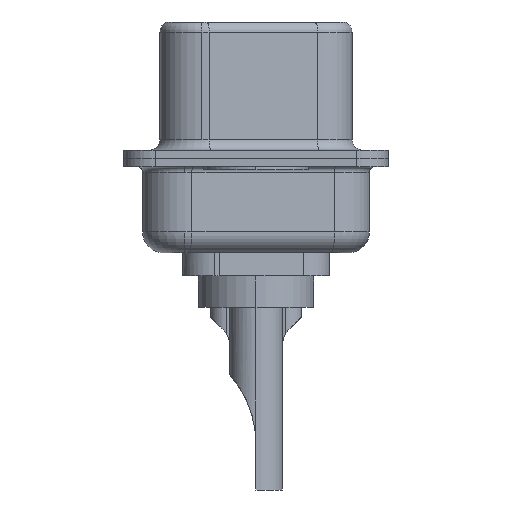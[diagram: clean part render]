
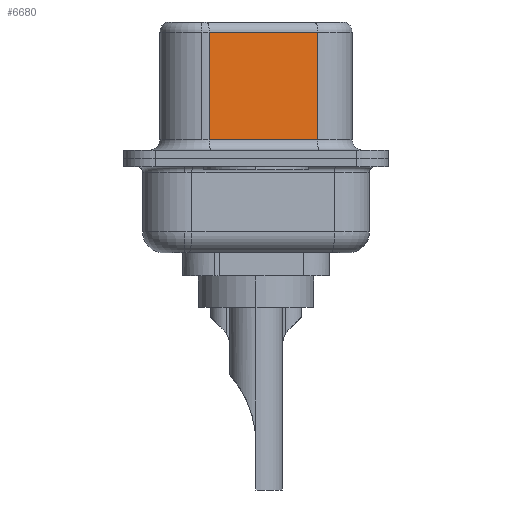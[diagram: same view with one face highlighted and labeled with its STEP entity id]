
A CAD part, left-side view. The second image highlights one B-rep face of the part: STEP entity #6680.
In plain terms, the highlighted planar face has unit normal (-0.985, -0.174, 0).
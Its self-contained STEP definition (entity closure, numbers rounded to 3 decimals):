
#112 = DIRECTION ( 'NONE',  ( 0.174, -0.985, 0. ) ) ;
#612 = DIRECTION ( 'NONE',  ( 0., 0., -1. ) ) ;
#1322 = CARTESIAN_POINT ( 'NONE',  ( 4.585, -2.927, 0.9 ) ) ;
#1980 = LINE ( 'NONE', #2978, #8455 ) ;
#2912 = DIRECTION ( 'NONE',  ( 0., 0., -1. ) ) ;
#2978 = CARTESIAN_POINT ( 'NONE',  ( 4.585, -2.927, 6.52 ) ) ;
#3822 = DIRECTION ( 'NONE',  ( -0.174, 0.985, 0. ) ) ;
#5234 = FACE_OUTER_BOUND ( 'NONE', #12017, .T. ) ;
#5388 = CARTESIAN_POINT ( 'NONE',  ( 3.675, 2.233, 6.52 ) ) ;
#5440 = ORIENTED_EDGE ( 'NONE', *, *, #6648, .T. ) ;
#6086 = VECTOR ( 'NONE', #3822, 1000. ) ;
#6648 = EDGE_CURVE ( 'NONE', #10150, #11646, #12345, .T. ) ;
#6673 = DIRECTION ( 'NONE',  ( 0.985, 0.174, 0. ) ) ;
#6680 = ADVANCED_FACE ( 'NONE', ( #5234 ), #11411, .F. ) ;
#6693 = EDGE_CURVE ( 'NONE', #13265, #9783, #1980, .T. ) ;
#7518 = CARTESIAN_POINT ( 'NONE',  ( 4.585, -2.927, 6.02 ) ) ;
#7602 = CARTESIAN_POINT ( 'NONE',  ( 4.585, -2.927, 0.9 ) ) ;
#8455 = VECTOR ( 'NONE', #612, 1000. ) ;
#9783 = VERTEX_POINT ( 'NONE', #7602 ) ;
#9978 = LINE ( 'NONE', #7518, #6086 ) ;
#10150 = VERTEX_POINT ( 'NONE', #14255 ) ;
#10217 = CARTESIAN_POINT ( 'NONE',  ( 4.585, -2.927, 6.52 ) ) ;
#10387 = ORIENTED_EDGE ( 'NONE', *, *, #6693, .F. ) ;
#10390 = ORIENTED_EDGE ( 'NONE', *, *, #12658, .T. ) ;
#10745 = ORIENTED_EDGE ( 'NONE', *, *, #11392, .T. ) ;
#11392 = EDGE_CURVE ( 'NONE', #11646, #9783, #13777, .T. ) ;
#11411 = PLANE ( 'NONE',  #14579 ) ;
#11542 = CARTESIAN_POINT ( 'NONE',  ( 4.585, -2.927, 6.02 ) ) ;
#11646 = VERTEX_POINT ( 'NONE', #15122 ) ;
#12017 = EDGE_LOOP ( 'NONE', ( #10387, #10390, #5440, #10745 ) ) ;
#12345 = LINE ( 'NONE', #5388, #14810 ) ;
#12658 = EDGE_CURVE ( 'NONE', #13265, #10150, #9978, .T. ) ;
#13265 = VERTEX_POINT ( 'NONE', #11542 ) ;
#13379 = VECTOR ( 'NONE', #112, 1000. ) ;
#13777 = LINE ( 'NONE', #1322, #13379 ) ;
#14255 = CARTESIAN_POINT ( 'NONE',  ( 3.675, 2.233, 6.02 ) ) ;
#14579 = AXIS2_PLACEMENT_3D ( 'NONE', #10217, #6673, #15037 ) ;
#14810 = VECTOR ( 'NONE', #2912, 1000. ) ;
#15037 = DIRECTION ( 'NONE',  ( -0.174, 0.985, 0. ) ) ;
#15122 = CARTESIAN_POINT ( 'NONE',  ( 3.675, 2.233, 0.9 ) ) ;
